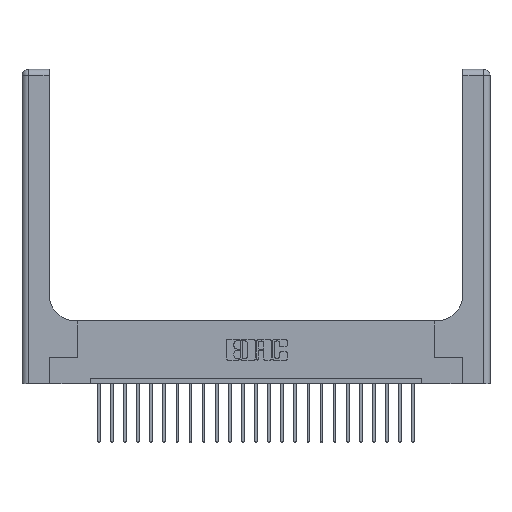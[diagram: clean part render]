
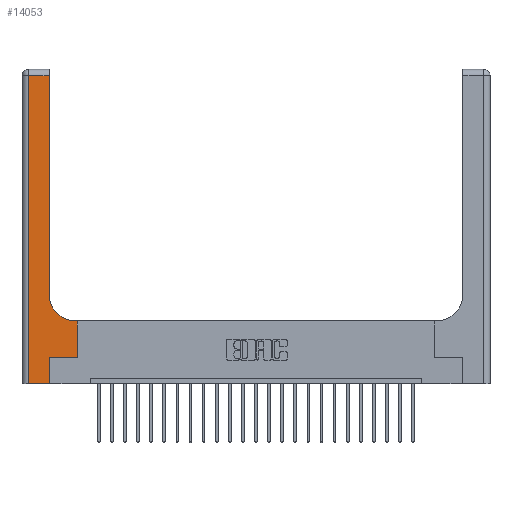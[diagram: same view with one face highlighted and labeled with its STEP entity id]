
A CAD part, top view. The second image highlights one B-rep face of the part: STEP entity #14053.
In plain terms, the highlighted planar face has unit normal (0, 0, 1).
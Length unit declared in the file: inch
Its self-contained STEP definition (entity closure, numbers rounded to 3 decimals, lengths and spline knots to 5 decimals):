
#18 = CARTESIAN_POINT ( 'NONE',  ( 0.265, 0., 0.37 ) ) ;
#548 = EDGE_CURVE ( 'NONE', #8253, #8045, #13372, .T. ) ;
#747 = CARTESIAN_POINT ( 'NONE',  ( 0.528, 0.6, 0.37 ) ) ;
#1038 = ORIENTED_EDGE ( 'NONE', *, *, #12825, .T. ) ;
#1169 = DIRECTION ( 'NONE',  ( 1., 0., 0. ) ) ;
#1277 = VERTEX_POINT ( 'NONE', #9940 ) ;
#1499 = VERTEX_POINT ( 'NONE', #19140 ) ;
#2556 = DIRECTION ( 'NONE',  ( -1., 0., 0. ) ) ;
#2635 = DIRECTION ( 'NONE',  ( 0., 0., -1. ) ) ;
#3442 = CARTESIAN_POINT ( 'NONE',  ( 0.06, 2.94, 0.37 ) ) ;
#4063 = VERTEX_POINT ( 'NONE', #747 ) ;
#4241 = AXIS2_PLACEMENT_3D ( 'NONE', #4692, #4541, #13545 ) ;
#4302 = CIRCLE ( 'NONE', #4241, 0.25 ) ;
#4460 = CARTESIAN_POINT ( 'NONE',  ( 0.265, 0.25, 0.37 ) ) ;
#4541 = DIRECTION ( 'NONE',  ( 0., 0., -1. ) ) ;
#4692 = CARTESIAN_POINT ( 'NONE',  ( 0.51, 0.85, 0.37 ) ) ;
#4741 = EDGE_LOOP ( 'NONE', ( #12890, #13497, #15031, #14317, #20930, #1038, #21245, #21119, #22570 ) ) ;
#5335 = DIRECTION ( 'NONE',  ( 0., 1., 0. ) ) ;
#5345 = CARTESIAN_POINT ( 'NONE',  ( 0.26, 2.94, 0.37 ) ) ;
#5680 = CARTESIAN_POINT ( 'NONE',  ( 0., 0., 0.37 ) ) ;
#5966 = EDGE_CURVE ( 'NONE', #4063, #1499, #13460, .T. ) ;
#6089 = EDGE_CURVE ( 'NONE', #1499, #8253, #4302, .T. ) ;
#6264 = PLANE ( 'NONE',  #21047 ) ;
#6493 = VERTEX_POINT ( 'NONE', #20152 ) ;
#7086 = FACE_OUTER_BOUND ( 'NONE', #4741, .T. ) ;
#7342 = CARTESIAN_POINT ( 'NONE',  ( 0.528, 0.25, 0.37 ) ) ;
#7557 = LINE ( 'NONE', #18, #10016 ) ;
#7616 = LINE ( 'NONE', #5680, #19597 ) ;
#7629 = LINE ( 'NONE', #7342, #11257 ) ;
#7741 = DIRECTION ( 'NONE',  ( -1., 0., 0. ) ) ;
#8045 = VERTEX_POINT ( 'NONE', #5345 ) ;
#8253 = VERTEX_POINT ( 'NONE', #10947 ) ;
#8384 = VECTOR ( 'NONE', #9406, 39.37008 ) ;
#8595 = VECTOR ( 'NONE', #5335, 39.37008 ) ;
#8711 = VECTOR ( 'NONE', #7741, 39.37008 ) ;
#8863 = DIRECTION ( 'NONE',  ( 0., 1., 0. ) ) ;
#9288 = VECTOR ( 'NONE', #13443, 39.37008 ) ;
#9310 = DIRECTION ( 'NONE',  ( 0., 1., 0. ) ) ;
#9406 = DIRECTION ( 'NONE',  ( -1., 0., 0. ) ) ;
#9600 = EDGE_CURVE ( 'NONE', #8045, #14641, #15075, .T. ) ;
#9679 = CARTESIAN_POINT ( 'NONE',  ( 0.26, 0.6, 0.37 ) ) ;
#9940 = CARTESIAN_POINT ( 'NONE',  ( 0.06, 0., 0.37 ) ) ;
#10016 = VECTOR ( 'NONE', #9310, 39.37008 ) ;
#10947 = CARTESIAN_POINT ( 'NONE',  ( 0.26, 0.85, 0.37 ) ) ;
#11019 = CARTESIAN_POINT ( 'NONE',  ( 0., 2.94, 0.37 ) ) ;
#11257 = VECTOR ( 'NONE', #8863, 39.37008 ) ;
#12324 = LINE ( 'NONE', #22403, #9288 ) ;
#12415 = CARTESIAN_POINT ( 'NONE',  ( 0.26, 3., 0.37 ) ) ;
#12825 = EDGE_CURVE ( 'NONE', #17159, #6493, #15509, .T. ) ;
#12890 = ORIENTED_EDGE ( 'NONE', *, *, #548, .T. ) ;
#13372 = LINE ( 'NONE', #12415, #8595 ) ;
#13443 = DIRECTION ( 'NONE',  ( 0., -1., 0. ) ) ;
#13460 = LINE ( 'NONE', #9679, #8711 ) ;
#13497 = ORIENTED_EDGE ( 'NONE', *, *, #9600, .T. ) ;
#13545 = DIRECTION ( 'NONE',  ( 1., 0., 0. ) ) ;
#13780 = VERTEX_POINT ( 'NONE', #17335 ) ;
#14053 = ADVANCED_FACE ( 'NONE', ( #7086 ), #6264, .F. ) ;
#14317 = ORIENTED_EDGE ( 'NONE', *, *, #16258, .T. ) ;
#14641 = VERTEX_POINT ( 'NONE', #3442 ) ;
#14762 = DIRECTION ( 'NONE',  ( 1., 0., 0. ) ) ;
#15031 = ORIENTED_EDGE ( 'NONE', *, *, #22551, .T. ) ;
#15075 = LINE ( 'NONE', #11019, #8384 ) ;
#15232 = EDGE_CURVE ( 'NONE', #6493, #4063, #7629, .T. ) ;
#15509 = LINE ( 'NONE', #4460, #17706 ) ;
#16258 = EDGE_CURVE ( 'NONE', #1277, #13780, #7616, .T. ) ;
#17159 = VERTEX_POINT ( 'NONE', #22366 ) ;
#17335 = CARTESIAN_POINT ( 'NONE',  ( 0.265, 0., 0.37 ) ) ;
#17582 = EDGE_CURVE ( 'NONE', #13780, #17159, #7557, .T. ) ;
#17706 = VECTOR ( 'NONE', #1169, 39.37008 ) ;
#18418 = CARTESIAN_POINT ( 'NONE',  ( 0., 3., 0.37 ) ) ;
#19140 = CARTESIAN_POINT ( 'NONE',  ( 0.51, 0.6, 0.37 ) ) ;
#19597 = VECTOR ( 'NONE', #14762, 39.37008 ) ;
#20152 = CARTESIAN_POINT ( 'NONE',  ( 0.528, 0.25, 0.37 ) ) ;
#20930 = ORIENTED_EDGE ( 'NONE', *, *, #17582, .T. ) ;
#21047 = AXIS2_PLACEMENT_3D ( 'NONE', #18418, #2635, #2556 ) ;
#21119 = ORIENTED_EDGE ( 'NONE', *, *, #5966, .T. ) ;
#21245 = ORIENTED_EDGE ( 'NONE', *, *, #15232, .T. ) ;
#22366 = CARTESIAN_POINT ( 'NONE',  ( 0.265, 0.25, 0.37 ) ) ;
#22403 = CARTESIAN_POINT ( 'NONE',  ( 0.06, 3., 0.37 ) ) ;
#22551 = EDGE_CURVE ( 'NONE', #14641, #1277, #12324, .T. ) ;
#22570 = ORIENTED_EDGE ( 'NONE', *, *, #6089, .T. ) ;
